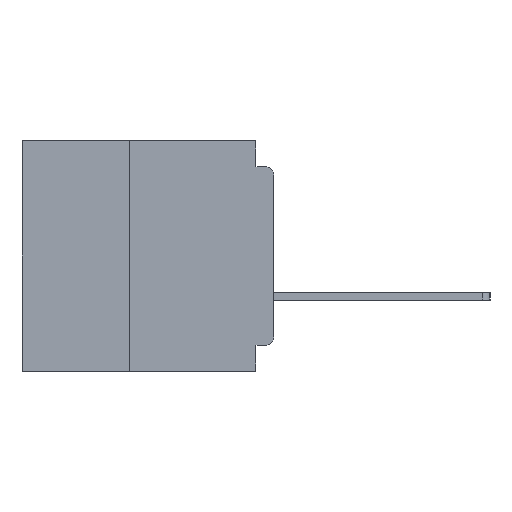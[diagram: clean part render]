
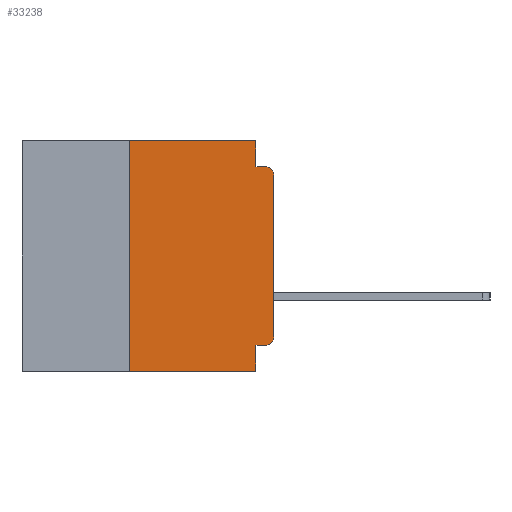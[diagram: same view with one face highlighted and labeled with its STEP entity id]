
A CAD part, left-side view. The second image highlights one B-rep face of the part: STEP entity #33238.
In plain terms, the highlighted planar face has unit normal (-1, 0, 0).
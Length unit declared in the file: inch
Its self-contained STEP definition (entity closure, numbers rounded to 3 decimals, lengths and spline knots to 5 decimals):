
#39 = VERTEX_POINT ( 'NONE', #31865 ) ;
#407 = DIRECTION ( 'NONE',  ( 0., 0., -1. ) ) ;
#473 = CARTESIAN_POINT ( 'NONE',  ( 0., 0.015, -0.34 ) ) ;
#576 = EDGE_CURVE ( 'NONE', #42977, #13441, #40957, .T. ) ;
#726 = DIRECTION ( 'NONE',  ( 0., 0., -1. ) ) ;
#2165 = CARTESIAN_POINT ( 'NONE',  ( 0., 0., 0. ) ) ;
#2389 = ORIENTED_EDGE ( 'NONE', *, *, #576, .T. ) ;
#2668 = CARTESIAN_POINT ( 'NONE',  ( 0., 0.25, -0.4 ) ) ;
#3746 = CARTESIAN_POINT ( 'NONE',  ( 0., 0., -0.045 ) ) ;
#4078 = DIRECTION ( 'NONE',  ( 0., 0., -1. ) ) ;
#6089 = CARTESIAN_POINT ( 'NONE',  ( 0., 0.25, 0. ) ) ;
#7221 = VECTOR ( 'NONE', #12818, 39.37008 ) ;
#7390 = LINE ( 'NONE', #28803, #41299 ) ;
#7597 = VERTEX_POINT ( 'NONE', #40206 ) ;
#8184 = CARTESIAN_POINT ( 'NONE',  ( 0., 0., -0.34 ) ) ;
#9577 = LINE ( 'NONE', #3746, #35352 ) ;
#10650 = VECTOR ( 'NONE', #23310, 39.37008 ) ;
#11083 = CARTESIAN_POINT ( 'NONE',  ( 0., 0.031, 0. ) ) ;
#11098 = LINE ( 'NONE', #24546, #28689 ) ;
#11939 = ORIENTED_EDGE ( 'NONE', *, *, #22465, .F. ) ;
#12818 = DIRECTION ( 'NONE',  ( 0., 0., 1. ) ) ;
#13441 = VERTEX_POINT ( 'NONE', #31802 ) ;
#14270 = CARTESIAN_POINT ( 'NONE',  ( 0., 0.25, -0.4 ) ) ;
#14582 = DIRECTION ( 'NONE',  ( 0., 0., -1. ) ) ;
#14790 = DIRECTION ( 'NONE',  ( 0., -1., 0. ) ) ;
#15774 = ORIENTED_EDGE ( 'NONE', *, *, #34488, .F. ) ;
#17228 = CARTESIAN_POINT ( 'NONE',  ( 0., 0.031, -0.4 ) ) ;
#17445 = CARTESIAN_POINT ( 'NONE',  ( 0., 0.437, 0. ) ) ;
#18860 = LINE ( 'NONE', #44141, #10650 ) ;
#18955 = ORIENTED_EDGE ( 'NONE', *, *, #33552, .T. ) ;
#19393 = LINE ( 'NONE', #25576, #32590 ) ;
#20416 = FACE_OUTER_BOUND ( 'NONE', #42278, .T. ) ;
#20994 = DIRECTION ( 'NONE',  ( 0., 0., -1. ) ) ;
#21150 = VECTOR ( 'NONE', #14582, 39.37008 ) ;
#21454 = CARTESIAN_POINT ( 'NONE',  ( 0., 0., -0.06 ) ) ;
#22251 = LINE ( 'NONE', #11083, #21150 ) ;
#22465 = EDGE_CURVE ( 'NONE', #39, #39507, #18860, .T. ) ;
#23310 = DIRECTION ( 'NONE',  ( 0., 1., 0. ) ) ;
#23442 = EDGE_CURVE ( 'NONE', #39507, #43449, #19393, .T. ) ;
#23457 = ORIENTED_EDGE ( 'NONE', *, *, #33280, .T. ) ;
#24381 = VERTEX_POINT ( 'NONE', #2668 ) ;
#24546 = CARTESIAN_POINT ( 'NONE',  ( 0., 0.437, -0.4 ) ) ;
#24735 = VECTOR ( 'NONE', #38778, 39.37008 ) ;
#25170 = DIRECTION ( 'NONE',  ( -1., 0., 0. ) ) ;
#25288 = CARTESIAN_POINT ( 'NONE',  ( 0., 0.015, -0.06 ) ) ;
#25576 = CARTESIAN_POINT ( 'NONE',  ( 0., 0.031, -0.4 ) ) ;
#27424 = EDGE_CURVE ( 'NONE', #29615, #13441, #9577, .T. ) ;
#27490 = EDGE_CURVE ( 'NONE', #40625, #7597, #7390, .T. ) ;
#28222 = ORIENTED_EDGE ( 'NONE', *, *, #27490, .F. ) ;
#28689 = VECTOR ( 'NONE', #38561, 39.37008 ) ;
#28803 = CARTESIAN_POINT ( 'NONE',  ( 0., 0.437, 0. ) ) ;
#29615 = VERTEX_POINT ( 'NONE', #41369 ) ;
#30200 = AXIS2_PLACEMENT_3D ( 'NONE', #473, #25170, #4078 ) ;
#31617 = ORIENTED_EDGE ( 'NONE', *, *, #27424, .F. ) ;
#31776 = EDGE_CURVE ( 'NONE', #7597, #29615, #22251, .T. ) ;
#31802 = CARTESIAN_POINT ( 'NONE',  ( 0., 0.015, -0.045 ) ) ;
#31865 = CARTESIAN_POINT ( 'NONE',  ( 0., 0.015, -0.355 ) ) ;
#32590 = VECTOR ( 'NONE', #726, 39.37008 ) ;
#32932 = ORIENTED_EDGE ( 'NONE', *, *, #35875, .T. ) ;
#32971 = ORIENTED_EDGE ( 'NONE', *, *, #31776, .F. ) ;
#33238 = ADVANCED_FACE ( 'NONE', ( #20416 ), #34767, .F. ) ;
#33280 = EDGE_CURVE ( 'NONE', #24381, #43449, #11098, .T. ) ;
#33552 = EDGE_CURVE ( 'NONE', #35842, #42977, #35198, .T. ) ;
#34255 = CARTESIAN_POINT ( 'NONE',  ( 0., 0.031, -0.355 ) ) ;
#34488 = EDGE_CURVE ( 'NONE', #24381, #40625, #41072, .T. ) ;
#34767 = PLANE ( 'NONE',  #35785 ) ;
#35198 = LINE ( 'NONE', #2165, #7221 ) ;
#35351 = DIRECTION ( 'NONE',  ( 0., -1., 0. ) ) ;
#35352 = VECTOR ( 'NONE', #35351, 39.37008 ) ;
#35608 = DIRECTION ( 'NONE',  ( -1., 0., 0. ) ) ;
#35785 = AXIS2_PLACEMENT_3D ( 'NONE', #17445, #41895, #20994 ) ;
#35842 = VERTEX_POINT ( 'NONE', #8184 ) ;
#35875 = EDGE_CURVE ( 'NONE', #39, #35842, #38876, .T. ) ;
#38561 = DIRECTION ( 'NONE',  ( 0., -1., 0. ) ) ;
#38778 = DIRECTION ( 'NONE',  ( 0., 0., 1. ) ) ;
#38876 = CIRCLE ( 'NONE', #30200, 0.015 ) ;
#39507 = VERTEX_POINT ( 'NONE', #34255 ) ;
#40206 = CARTESIAN_POINT ( 'NONE',  ( 0., 0.031, 0. ) ) ;
#40625 = VERTEX_POINT ( 'NONE', #6089 ) ;
#40957 = CIRCLE ( 'NONE', #45243, 0.015 ) ;
#41072 = LINE ( 'NONE', #14270, #24735 ) ;
#41299 = VECTOR ( 'NONE', #14790, 39.37008 ) ;
#41369 = CARTESIAN_POINT ( 'NONE',  ( 0., 0.031, -0.045 ) ) ;
#41895 = DIRECTION ( 'NONE',  ( 1., 0., 0. ) ) ;
#42278 = EDGE_LOOP ( 'NONE', ( #18955, #2389, #31617, #32971, #28222, #15774, #23457, #43212, #11939, #32932 ) ) ;
#42977 = VERTEX_POINT ( 'NONE', #21454 ) ;
#43212 = ORIENTED_EDGE ( 'NONE', *, *, #23442, .F. ) ;
#43449 = VERTEX_POINT ( 'NONE', #17228 ) ;
#44141 = CARTESIAN_POINT ( 'NONE',  ( 0., 0., -0.355 ) ) ;
#45243 = AXIS2_PLACEMENT_3D ( 'NONE', #25288, #35608, #407 ) ;
